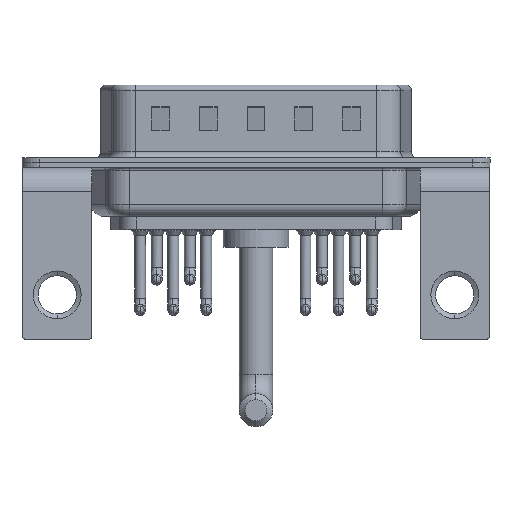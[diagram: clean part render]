
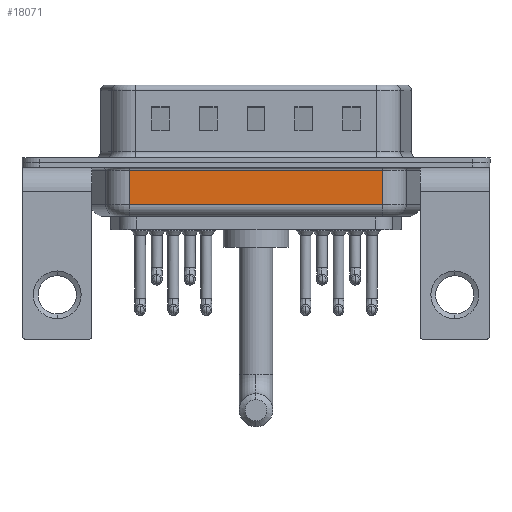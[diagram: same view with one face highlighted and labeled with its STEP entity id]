
A CAD part, front view. The second image highlights one B-rep face of the part: STEP entity #18071.
In plain terms, the highlighted planar face has unit normal (0, -1, 0).
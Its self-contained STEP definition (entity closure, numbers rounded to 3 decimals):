
#13 = VECTOR ( 'NONE', #8565, 1000. ) ;
#963 = ORIENTED_EDGE ( 'NONE', *, *, #22555, .F. ) ;
#1840 = CARTESIAN_POINT ( 'NONE',  ( 6.031, -5.35, -4.5 ) ) ;
#2937 = ORIENTED_EDGE ( 'NONE', *, *, #11235, .T. ) ;
#2960 = ORIENTED_EDGE ( 'NONE', *, *, #21599, .T. ) ;
#3611 = DIRECTION ( 'NONE',  ( 0., 1., 0. ) ) ;
#5182 = VECTOR ( 'NONE', #19692, 1000. ) ;
#5195 = CARTESIAN_POINT ( 'NONE',  ( 6.031, -5.35, -0.65 ) ) ;
#6265 = VERTEX_POINT ( 'NONE', #16363 ) ;
#7215 = CARTESIAN_POINT ( 'NONE',  ( 6.031, -5.35, -0.65 ) ) ;
#7301 = LINE ( 'NONE', #14481, #5182 ) ;
#7306 = LINE ( 'NONE', #11051, #16136 ) ;
#8386 = EDGE_LOOP ( 'NONE', ( #963, #2960, #2937, #22742 ) ) ;
#8565 = DIRECTION ( 'NONE',  ( 0., 0., 1. ) ) ;
#10320 = CARTESIAN_POINT ( 'NONE',  ( 6.031, -5.35, -4.5 ) ) ;
#11051 = CARTESIAN_POINT ( 'NONE',  ( 6.031, -5.35, -3.5 ) ) ;
#11235 = EDGE_CURVE ( 'NONE', #14892, #6265, #7301, .T. ) ;
#12110 = VERTEX_POINT ( 'NONE', #5195 ) ;
#12407 = DIRECTION ( 'NONE',  ( 0., 0., 1. ) ) ;
#13616 = FACE_OUTER_BOUND ( 'NONE', #8386, .T. ) ;
#14065 = PLANE ( 'NONE',  #22467 ) ;
#14481 = CARTESIAN_POINT ( 'NONE',  ( 27.269, -5.35, -4.5 ) ) ;
#14892 = VERTEX_POINT ( 'NONE', #20482 ) ;
#15927 = DIRECTION ( 'NONE',  ( -1., 0., 0. ) ) ;
#16136 = VECTOR ( 'NONE', #19816, 1000. ) ;
#16363 = CARTESIAN_POINT ( 'NONE',  ( 27.269, -5.35, -0.65 ) ) ;
#18071 = ADVANCED_FACE ( 'NONE', ( #13616 ), #14065, .F. ) ;
#18281 = LINE ( 'NONE', #7215, #20272 ) ;
#18638 = CARTESIAN_POINT ( 'NONE',  ( 6.031, -5.35, -3.5 ) ) ;
#19692 = DIRECTION ( 'NONE',  ( 0., 0., 1. ) ) ;
#19816 = DIRECTION ( 'NONE',  ( 1., 0., 0. ) ) ;
#20272 = VECTOR ( 'NONE', #15927, 1000. ) ;
#20482 = CARTESIAN_POINT ( 'NONE',  ( 27.269, -5.35, -3.5 ) ) ;
#20743 = EDGE_CURVE ( 'NONE', #6265, #12110, #18281, .T. ) ;
#21453 = VERTEX_POINT ( 'NONE', #18638 ) ;
#21599 = EDGE_CURVE ( 'NONE', #21453, #14892, #7306, .T. ) ;
#22467 = AXIS2_PLACEMENT_3D ( 'NONE', #1840, #3611, #12407 ) ;
#22555 = EDGE_CURVE ( 'NONE', #21453, #12110, #23329, .T. ) ;
#22742 = ORIENTED_EDGE ( 'NONE', *, *, #20743, .T. ) ;
#23329 = LINE ( 'NONE', #10320, #13 ) ;
